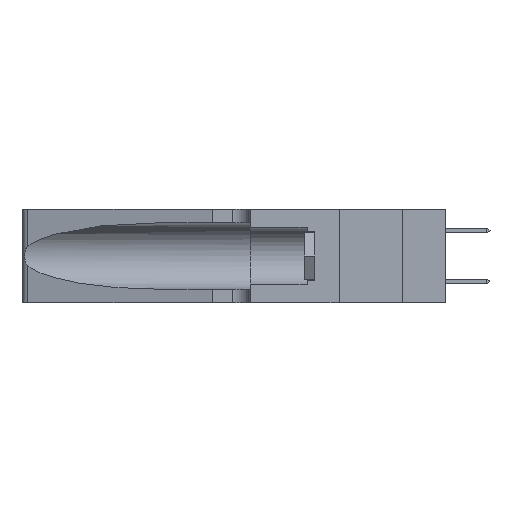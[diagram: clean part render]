
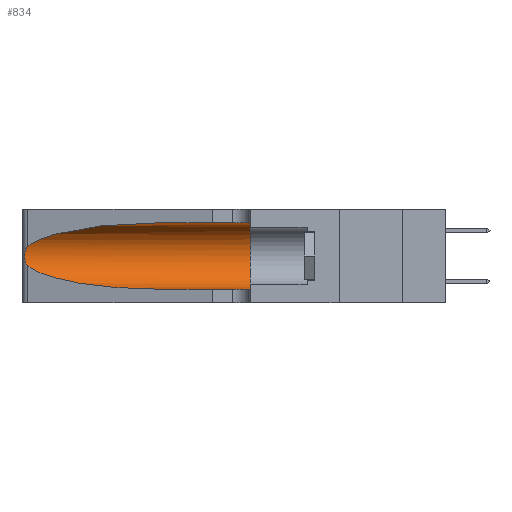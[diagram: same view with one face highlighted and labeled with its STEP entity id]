
A CAD part, left-side view. The second image highlights one B-rep face of the part: STEP entity #834.
In plain terms, the highlighted cylindrical face has radius 3.308 mm (diameter 6.617 mm), a partial arc.
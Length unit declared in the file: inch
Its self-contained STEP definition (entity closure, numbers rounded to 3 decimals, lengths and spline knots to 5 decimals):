
#528 = CARTESIAN_POINT ( 'NONE',  ( 0.1305, 0.35, 0.31525 ) ) ;
#660 = FACE_OUTER_BOUND ( 'NONE', #10718, .T. ) ;
#834 = ADVANCED_FACE ( 'NONE', ( #660 ), #8511, .F. ) ;
#1257 = ORIENTED_EDGE ( 'NONE', *, *, #8931, .F. ) ;
#1335 = CARTESIAN_POINT ( 'NONE',  ( 0.26017, 1.23833, 0.17102 ) ) ;
#2879 = CARTESIAN_POINT ( 'NONE',  ( 0.26018, 1.23835, 0.19895 ) ) ;
#2910 = CARTESIAN_POINT ( 'NONE',  ( 0.25487, 1.22718, 0.14631 ) ) ;
#3010 = CARTESIAN_POINT ( 'NONE',  ( 0.2373, 1.15595, 0.28018 ) ) ;
#3159 = DIRECTION ( 'NONE',  ( 0., 0., -1. ) ) ;
#3849 = VERTEX_POINT ( 'NONE', #4427 ) ;
#4427 = CARTESIAN_POINT ( 'NONE',  ( 0.1305, 0.72297, 0.05475 ) ) ;
#4705 = CARTESIAN_POINT ( 'NONE',  ( 0.1305, 0.35, 0.185 ) ) ;
#6222 = CARTESIAN_POINT ( 'NONE',  ( 0.1305, 0.72297, 0.31525 ) ) ;
#6267 = CARTESIAN_POINT ( 'NONE',  ( 0.1305, 0.72297, 0.05475 ) ) ;
#6310 = VECTOR ( 'NONE', #17512, 39.37008 ) ;
#6432 = CARTESIAN_POINT ( 'NONE',  ( 0.18966, 0.96281, 0.31525 ) ) ;
#6444 = CARTESIAN_POINT ( 'NONE',  ( 0.25789, 1.23486, 0.15765 ) ) ;
#6550 = LINE ( 'NONE', #7567, #6310 ) ;
#7186 = VERTEX_POINT ( 'NONE', #528 ) ;
#7567 = CARTESIAN_POINT ( 'NONE',  ( 0.1305, 1.61858, 0.05475 ) ) ;
#7981 = VERTEX_POINT ( 'NONE', #20192 ) ;
#8378 = EDGE_CURVE ( 'NONE', #3849, #17519, #6550, .T. ) ;
#8511 = CYLINDRICAL_SURFACE ( 'NONE', #19314, 0.13025 ) ;
#8561 = CARTESIAN_POINT ( 'NONE',  ( 0.25487, 1.22718, 0.14631 ) ) ;
#8931 = EDGE_CURVE ( 'NONE', #7186, #17519, #9962, .T. ) ;
#9159 = B_SPLINE_CURVE_WITH_KNOTS ( 'NONE', 3,
 ( #15599, #18970, #16187, #18031, #11309, #2879, #11668, #16690, #1335, #14722, #6444, #14877, #10321, #8561 ),
 .UNSPECIFIED., .F., .F.,
 ( 4, 2, 2, 2, 2, 2, 4 ),
 ( 0., 0.00027, 0.00053, 0.00107, 0.0016, 0.00187, 0.00214 ),
 .UNSPECIFIED. ) ;
#9848 = ORIENTED_EDGE ( 'NONE', *, *, #17711, .T. ) ;
#9962 = CIRCLE ( 'NONE', #14008, 0.13025 ) ;
#10027 = DIRECTION ( 'NONE',  ( 0., -1., 0. ) ) ;
#10321 = CARTESIAN_POINT ( 'NONE',  ( 0.25555, 1.22993, 0.14849 ) ) ;
#10718 = EDGE_LOOP ( 'NONE', ( #9848, #21061, #21104, #14236, #1257, #21013 ) ) ;
#11309 = CARTESIAN_POINT ( 'NONE',  ( 0.25854, 1.2359, 0.20912 ) ) ;
#11668 = CARTESIAN_POINT ( 'NONE',  ( 0.26075, 1.23896, 0.19203 ) ) ;
#11860 = CARTESIAN_POINT ( 'NONE',  ( 0.1305, 1.61858, 0.185 ) ) ;
#11959 = VECTOR ( 'NONE', #13627, 39.37008 ) ;
#12552 = EDGE_CURVE ( 'NONE', #7981, #18891, #9159, .T. ) ;
#12633 =( BOUNDED_CURVE ( )  B_SPLINE_CURVE ( 3, ( #2910, #19586, #14616, #6267 ),
 .UNSPECIFIED., .F., .F. ) 
 B_SPLINE_CURVE_WITH_KNOTS ( ( 4, 4 ),
 ( 3.44316, 4.71239 ),
 .UNSPECIFIED. ) 
 CURVE ( )  GEOMETRIC_REPRESENTATION_ITEM ( )  RATIONAL_B_SPLINE_CURVE ( ( 1., 0.87, 0.87, 1. ) ) 
 REPRESENTATION_ITEM ( '' )  );
#13627 = DIRECTION ( 'NONE',  ( 0., -1., 0. ) ) ;
#14008 = AXIS2_PLACEMENT_3D ( 'NONE', #4705, #16121, #16260 ) ;
#14236 = ORIENTED_EDGE ( 'NONE', *, *, #8378, .T. ) ;
#14265 = EDGE_CURVE ( 'NONE', #18891, #3849, #12633, .T. ) ;
#14270 = CARTESIAN_POINT ( 'NONE',  ( 0.25487, 1.22718, 0.14631 ) ) ;
#14616 = CARTESIAN_POINT ( 'NONE',  ( 0.18966, 0.96281, 0.05475 ) ) ;
#14722 = CARTESIAN_POINT ( 'NONE',  ( 0.25856, 1.23593, 0.16098 ) ) ;
#14877 = CARTESIAN_POINT ( 'NONE',  ( 0.25639, 1.23186, 0.15144 ) ) ;
#15599 = CARTESIAN_POINT ( 'NONE',  ( 0.25487, 1.22718, 0.22369 ) ) ;
#16093 = EDGE_CURVE ( 'NONE', #17222, #7186, #19031, .T. ) ;
#16121 = DIRECTION ( 'NONE',  ( 0., 1., 0. ) ) ;
#16187 = CARTESIAN_POINT ( 'NONE',  ( 0.25639, 1.23184, 0.21858 ) ) ;
#16260 = DIRECTION ( 'NONE',  ( 0., 0., 1. ) ) ;
#16690 = CARTESIAN_POINT ( 'NONE',  ( 0.26075, 1.23896, 0.178 ) ) ;
#17222 = VERTEX_POINT ( 'NONE', #19660 ) ;
#17512 = DIRECTION ( 'NONE',  ( 0., -1., 0. ) ) ;
#17519 = VERTEX_POINT ( 'NONE', #18958 ) ;
#17711 = EDGE_CURVE ( 'NONE', #17222, #7981, #21678, .T. ) ;
#17934 = CARTESIAN_POINT ( 'NONE',  ( 0.25487, 1.22718, 0.22369 ) ) ;
#18031 = CARTESIAN_POINT ( 'NONE',  ( 0.25787, 1.23484, 0.2124 ) ) ;
#18891 = VERTEX_POINT ( 'NONE', #14270 ) ;
#18958 = CARTESIAN_POINT ( 'NONE',  ( 0.1305, 0.35, 0.05475 ) ) ;
#18970 = CARTESIAN_POINT ( 'NONE',  ( 0.25555, 1.22994, 0.2215 ) ) ;
#19031 = LINE ( 'NONE', #20339, #11959 ) ;
#19314 = AXIS2_PLACEMENT_3D ( 'NONE', #11860, #10027, #3159 ) ;
#19586 = CARTESIAN_POINT ( 'NONE',  ( 0.2373, 1.15595, 0.08982 ) ) ;
#19660 = CARTESIAN_POINT ( 'NONE',  ( 0.1305, 0.72297, 0.31525 ) ) ;
#20192 = CARTESIAN_POINT ( 'NONE',  ( 0.25487, 1.22718, 0.22369 ) ) ;
#20339 = CARTESIAN_POINT ( 'NONE',  ( 0.1305, 1.61858, 0.31525 ) ) ;
#21013 = ORIENTED_EDGE ( 'NONE', *, *, #16093, .F. ) ;
#21061 = ORIENTED_EDGE ( 'NONE', *, *, #12552, .T. ) ;
#21104 = ORIENTED_EDGE ( 'NONE', *, *, #14265, .T. ) ;
#21678 =( BOUNDED_CURVE ( )  B_SPLINE_CURVE ( 3, ( #6222, #6432, #3010, #17934 ),
 .UNSPECIFIED., .F., .T. ) 
 B_SPLINE_CURVE_WITH_KNOTS ( ( 4, 4 ),
 ( 1.5708, 2.84003 ),
 .UNSPECIFIED. ) 
 CURVE ( )  GEOMETRIC_REPRESENTATION_ITEM ( )  RATIONAL_B_SPLINE_CURVE ( ( 1., 0.87, 0.87, 1. ) ) 
 REPRESENTATION_ITEM ( '' )  );
